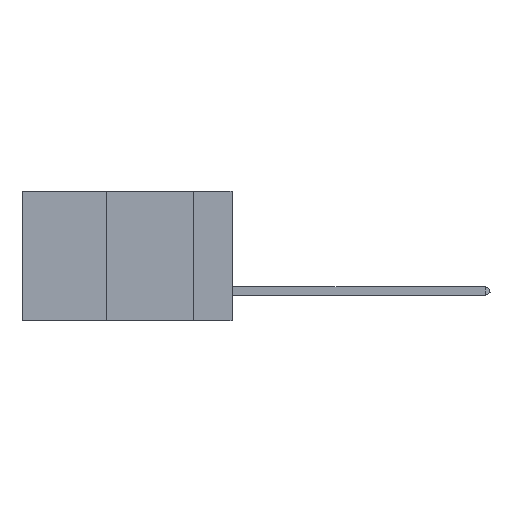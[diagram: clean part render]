
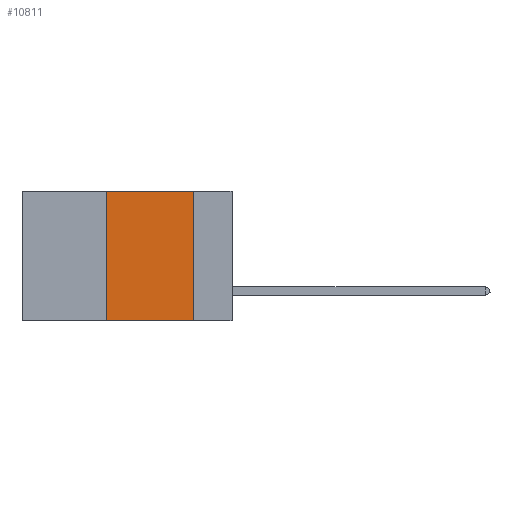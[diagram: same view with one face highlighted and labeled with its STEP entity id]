
A CAD part, left-side view. The second image highlights one B-rep face of the part: STEP entity #10811.
In plain terms, the highlighted planar face has unit normal (-1, 0, 0).
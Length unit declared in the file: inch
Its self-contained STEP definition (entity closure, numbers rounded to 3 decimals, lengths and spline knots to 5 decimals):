
#233 = LINE ( 'NONE', #2920, #1651 ) ;
#622 = EDGE_CURVE ( 'NONE', #1419, #9292, #233, .T. ) ;
#784 = VERTEX_POINT ( 'NONE', #9749 ) ;
#1419 = VERTEX_POINT ( 'NONE', #12364 ) ;
#1470 = CARTESIAN_POINT ( 'NONE',  ( 0., 0.6, 0. ) ) ;
#1651 = VECTOR ( 'NONE', #4429, 39.37008 ) ;
#2407 = VECTOR ( 'NONE', #13148, 39.37008 ) ;
#2920 = CARTESIAN_POINT ( 'NONE',  ( 0., 0.11, 0. ) ) ;
#4092 = CARTESIAN_POINT ( 'NONE',  ( 0., 0.11, -0.37 ) ) ;
#4429 = DIRECTION ( 'NONE',  ( 0., 0., -1. ) ) ;
#5487 = DIRECTION ( 'NONE',  ( 0., -1., 0. ) ) ;
#5609 = CARTESIAN_POINT ( 'NONE',  ( 0., 0.36, -0.37 ) ) ;
#5762 = CARTESIAN_POINT ( 'NONE',  ( 0., 0.36, 0. ) ) ;
#5822 = DIRECTION ( 'NONE',  ( 0., 0., 1. ) ) ;
#6036 = EDGE_CURVE ( 'NONE', #8509, #784, #10358, .T. ) ;
#6787 = EDGE_LOOP ( 'NONE', ( #13311, #11789, #16049, #10598 ) ) ;
#6802 = FACE_OUTER_BOUND ( 'NONE', #6787, .T. ) ;
#8067 = LINE ( 'NONE', #1470, #2407 ) ;
#8251 = AXIS2_PLACEMENT_3D ( 'NONE', #11100, #13712, #16447 ) ;
#8320 = LINE ( 'NONE', #10593, #8914 ) ;
#8509 = VERTEX_POINT ( 'NONE', #5609 ) ;
#8914 = VECTOR ( 'NONE', #5487, 39.37008 ) ;
#9292 = VERTEX_POINT ( 'NONE', #4092 ) ;
#9749 = CARTESIAN_POINT ( 'NONE',  ( 0., 0.36, 0. ) ) ;
#10358 = LINE ( 'NONE', #5762, #11170 ) ;
#10593 = CARTESIAN_POINT ( 'NONE',  ( 0., 0.6, -0.37 ) ) ;
#10598 = ORIENTED_EDGE ( 'NONE', *, *, #13246, .T. ) ;
#10811 = ADVANCED_FACE ( 'NONE', ( #6802 ), #16206, .F. ) ;
#11100 = CARTESIAN_POINT ( 'NONE',  ( 0., 0.6, 0. ) ) ;
#11170 = VECTOR ( 'NONE', #5822, 39.37008 ) ;
#11789 = ORIENTED_EDGE ( 'NONE', *, *, #14613, .F. ) ;
#12364 = CARTESIAN_POINT ( 'NONE',  ( 0., 0.11, 0. ) ) ;
#13148 = DIRECTION ( 'NONE',  ( 0., -1., 0. ) ) ;
#13246 = EDGE_CURVE ( 'NONE', #8509, #9292, #8320, .T. ) ;
#13311 = ORIENTED_EDGE ( 'NONE', *, *, #622, .F. ) ;
#13712 = DIRECTION ( 'NONE',  ( 1., 0., 0. ) ) ;
#14613 = EDGE_CURVE ( 'NONE', #784, #1419, #8067, .T. ) ;
#16049 = ORIENTED_EDGE ( 'NONE', *, *, #6036, .F. ) ;
#16206 = PLANE ( 'NONE',  #8251 ) ;
#16447 = DIRECTION ( 'NONE',  ( 0., 0., -1. ) ) ;
